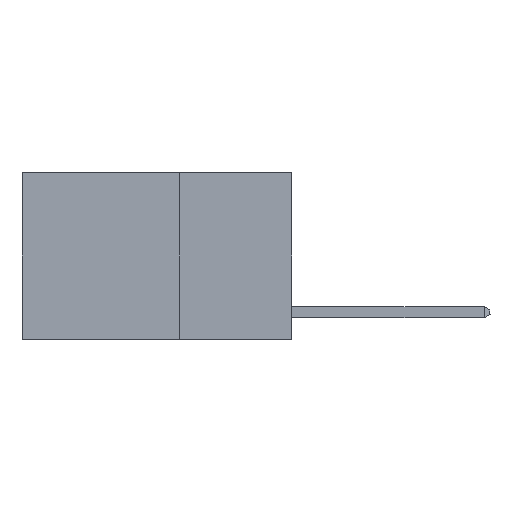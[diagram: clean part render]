
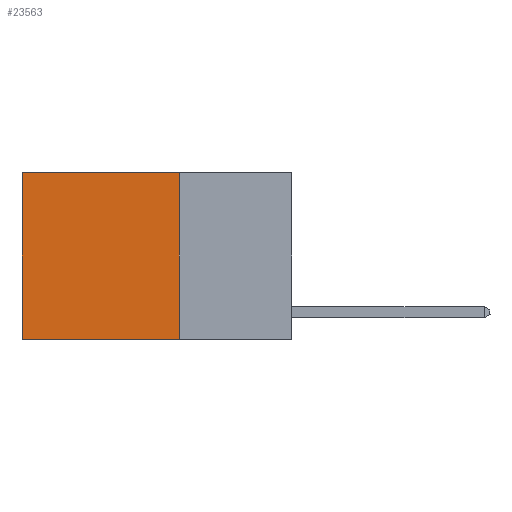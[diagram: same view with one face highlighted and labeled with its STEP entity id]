
A CAD part, left-side view. The second image highlights one B-rep face of the part: STEP entity #23563.
In plain terms, the highlighted planar face has unit normal (-1, 0, 0).
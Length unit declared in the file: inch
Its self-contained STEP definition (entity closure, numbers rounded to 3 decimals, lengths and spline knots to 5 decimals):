
#181 = CARTESIAN_POINT ( 'NONE',  ( 0.2625, 0.25, -0.37 ) ) ;
#781 = VECTOR ( 'NONE', #8011, 39.37008 ) ;
#2309 = CARTESIAN_POINT ( 'NONE',  ( 0.2625, 0.25, 0. ) ) ;
#3117 = CARTESIAN_POINT ( 'NONE',  ( 0.2625, 0.6, -0.37 ) ) ;
#3124 = VERTEX_POINT ( 'NONE', #181 ) ;
#4292 = ORIENTED_EDGE ( 'NONE', *, *, #20822, .F. ) ;
#4459 = DIRECTION ( 'NONE',  ( 0., 0., -1. ) ) ;
#4634 = PLANE ( 'NONE',  #13283 ) ;
#5818 = EDGE_CURVE ( 'NONE', #3124, #20185, #18452, .T. ) ;
#6934 = CARTESIAN_POINT ( 'NONE',  ( 0.2625, 0.25, -0.37 ) ) ;
#7852 = ORIENTED_EDGE ( 'NONE', *, *, #5818, .F. ) ;
#8011 = DIRECTION ( 'NONE',  ( 0., 1., 0. ) ) ;
#8143 = LINE ( 'NONE', #15965, #8782 ) ;
#8521 = EDGE_LOOP ( 'NONE', ( #20828, #7852, #4292, #23631 ) ) ;
#8782 = VECTOR ( 'NONE', #4459, 39.37008 ) ;
#9441 = CARTESIAN_POINT ( 'NONE',  ( 0.2625, 0.6, 0. ) ) ;
#9910 = EDGE_CURVE ( 'NONE', #14442, #20185, #8143, .T. ) ;
#11196 = DIRECTION ( 'NONE',  ( 0., 0., -1. ) ) ;
#12264 = LINE ( 'NONE', #24044, #15671 ) ;
#12343 = CARTESIAN_POINT ( 'NONE',  ( 0.2625, 0.25, 0. ) ) ;
#13283 = AXIS2_PLACEMENT_3D ( 'NONE', #12343, #20078, #11196 ) ;
#13948 = LINE ( 'NONE', #2309, #781 ) ;
#14442 = VERTEX_POINT ( 'NONE', #9441 ) ;
#14661 = DIRECTION ( 'NONE',  ( 0., 1., 0. ) ) ;
#15671 = VECTOR ( 'NONE', #19998, 39.37008 ) ;
#15965 = CARTESIAN_POINT ( 'NONE',  ( 0.2625, 0.6, 0. ) ) ;
#17496 = VECTOR ( 'NONE', #14661, 39.37008 ) ;
#18452 = LINE ( 'NONE', #6934, #17496 ) ;
#18545 = VERTEX_POINT ( 'NONE', #24660 ) ;
#19998 = DIRECTION ( 'NONE',  ( 0., 0., -1. ) ) ;
#20078 = DIRECTION ( 'NONE',  ( 1., 0., 0. ) ) ;
#20185 = VERTEX_POINT ( 'NONE', #3117 ) ;
#20822 = EDGE_CURVE ( 'NONE', #18545, #3124, #12264, .T. ) ;
#20828 = ORIENTED_EDGE ( 'NONE', *, *, #9910, .T. ) ;
#21994 = FACE_OUTER_BOUND ( 'NONE', #8521, .T. ) ;
#22904 = EDGE_CURVE ( 'NONE', #18545, #14442, #13948, .T. ) ;
#23563 = ADVANCED_FACE ( 'NONE', ( #21994 ), #4634, .F. ) ;
#23631 = ORIENTED_EDGE ( 'NONE', *, *, #22904, .T. ) ;
#24044 = CARTESIAN_POINT ( 'NONE',  ( 0.2625, 0.25, 0. ) ) ;
#24660 = CARTESIAN_POINT ( 'NONE',  ( 0.2625, 0.25, 0. ) ) ;
